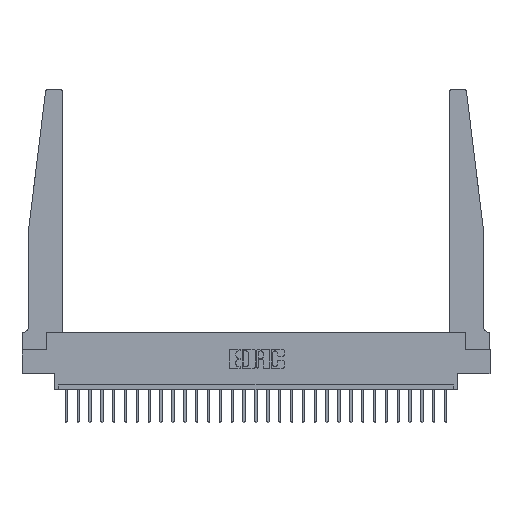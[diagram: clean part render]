
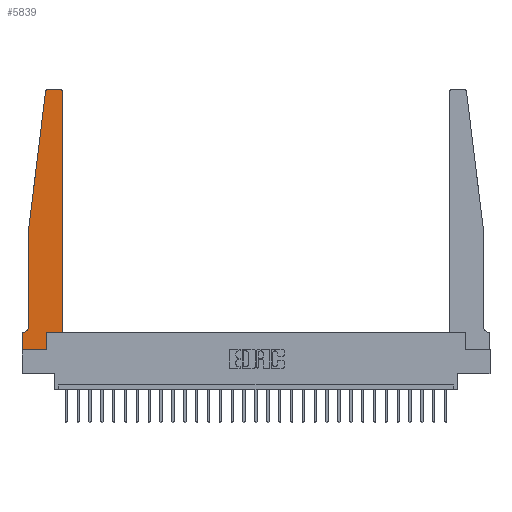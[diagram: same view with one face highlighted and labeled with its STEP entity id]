
A CAD part, top view. The second image highlights one B-rep face of the part: STEP entity #5839.
In plain terms, the highlighted planar face has unit normal (0, 0, 1).
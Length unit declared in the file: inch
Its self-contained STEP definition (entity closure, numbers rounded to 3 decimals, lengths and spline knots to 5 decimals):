
#637 = VERTEX_POINT ( 'NONE', #10416 ) ;
#946 = VERTEX_POINT ( 'NONE', #3312 ) ;
#1009 = CARTESIAN_POINT ( 'NONE',  ( 0.425, 0.18, 0.37 ) ) ;
#1124 = AXIS2_PLACEMENT_3D ( 'NONE', #7279, #9356, #19669 ) ;
#1316 = LINE ( 'NONE', #21824, #3554 ) ;
#1574 = DIRECTION ( 'NONE',  ( -1., 0., 0. ) ) ;
#1667 = EDGE_CURVE ( 'NONE', #16002, #22770, #25779, .T. ) ;
#1725 = CARTESIAN_POINT ( 'NONE',  ( 0., 0., 0.37 ) ) ;
#1814 = CARTESIAN_POINT ( 'NONE',  ( 0.2605, 0.18, 0.37 ) ) ;
#1879 = CARTESIAN_POINT ( 'NONE',  ( 0.27653, 2.75, 0.37 ) ) ;
#2254 = AXIS2_PLACEMENT_3D ( 'NONE', #18220, #24083, #1574 ) ;
#3105 = ORIENTED_EDGE ( 'NONE', *, *, #24069, .T. ) ;
#3312 = CARTESIAN_POINT ( 'NONE',  ( 0., 0.1875, 0.37 ) ) ;
#3509 = CIRCLE ( 'NONE', #10659, 0.03 ) ;
#3554 = VECTOR ( 'NONE', #13982, 39.37008 ) ;
#3640 = CARTESIAN_POINT ( 'NONE',  ( 0.065, 1.25, 0.37 ) ) ;
#3657 = VECTOR ( 'NONE', #10116, 39.37008 ) ;
#4074 = VECTOR ( 'NONE', #10125, 39.37008 ) ;
#4075 = CARTESIAN_POINT ( 'NONE',  ( 0.395, 2.75, 0.37 ) ) ;
#4081 = DIRECTION ( 'NONE',  ( 0., -1., 0. ) ) ;
#4325 = ORIENTED_EDGE ( 'NONE', *, *, #22656, .T. ) ;
#4931 = EDGE_CURVE ( 'NONE', #637, #23798, #25307, .T. ) ;
#5839 = ADVANCED_FACE ( 'NONE', ( #18187 ), #21760, .T. ) ;
#6051 = LINE ( 'NONE', #3640, #24047 ) ;
#6699 = VERTEX_POINT ( 'NONE', #6936 ) ;
#6936 = CARTESIAN_POINT ( 'NONE',  ( 0., 0., 0.37 ) ) ;
#7279 = CARTESIAN_POINT ( 'NONE',  ( 0., 0.1875, 0.37 ) ) ;
#7726 = DIRECTION ( 'NONE',  ( -0.122, -0.992, 0. ) ) ;
#7737 = AXIS2_PLACEMENT_3D ( 'NONE', #23165, #12834, #21101 ) ;
#8115 = ORIENTED_EDGE ( 'NONE', *, *, #17398, .T. ) ;
#8948 = VECTOR ( 'NONE', #19988, 39.37008 ) ;
#9356 = DIRECTION ( 'NONE',  ( 0., 0., 1. ) ) ;
#9669 = CARTESIAN_POINT ( 'NONE',  ( 0.2605, 0.18, 0.37 ) ) ;
#10116 = DIRECTION ( 'NONE',  ( 1., 0., 0. ) ) ;
#10125 = DIRECTION ( 'NONE',  ( 1., 0., 0. ) ) ;
#10416 = CARTESIAN_POINT ( 'NONE',  ( 0.2605, 0., 0.37 ) ) ;
#10659 = AXIS2_PLACEMENT_3D ( 'NONE', #15526, #17858, #11392 ) ;
#10714 = DIRECTION ( 'NONE',  ( 0., -1., 0. ) ) ;
#11392 = DIRECTION ( 'NONE',  ( 1., 0., 0. ) ) ;
#11589 = EDGE_CURVE ( 'NONE', #946, #6699, #17667, .T. ) ;
#12619 = EDGE_CURVE ( 'NONE', #6699, #637, #15049, .T. ) ;
#12621 = LINE ( 'NONE', #21473, #13282 ) ;
#12629 = ORIENTED_EDGE ( 'NONE', *, *, #1667, .T. ) ;
#12646 = VERTEX_POINT ( 'NONE', #4075 ) ;
#12834 = DIRECTION ( 'NONE',  ( 0., 0., 1. ) ) ;
#13282 = VECTOR ( 'NONE', #25388, 39.37008 ) ;
#13333 = ORIENTED_EDGE ( 'NONE', *, *, #25002, .T. ) ;
#13612 = ORIENTED_EDGE ( 'NONE', *, *, #12619, .T. ) ;
#13982 = DIRECTION ( 'NONE',  ( -1., 0., 0. ) ) ;
#14077 = CARTESIAN_POINT ( 'NONE',  ( 0.425, 2.72, 0.37 ) ) ;
#14176 = CARTESIAN_POINT ( 'NONE',  ( 0.24675, 2.72367, 0.37 ) ) ;
#14273 = VECTOR ( 'NONE', #19363, 39.37008 ) ;
#15049 = LINE ( 'NONE', #1725, #4074 ) ;
#15171 = VERTEX_POINT ( 'NONE', #1879 ) ;
#15319 = ORIENTED_EDGE ( 'NONE', *, *, #11589, .T. ) ;
#15526 = CARTESIAN_POINT ( 'NONE',  ( 0.27653, 2.72, 0.37 ) ) ;
#15672 = EDGE_CURVE ( 'NONE', #12646, #15171, #24545, .T. ) ;
#16002 = VERTEX_POINT ( 'NONE', #24972 ) ;
#16505 = EDGE_CURVE ( 'NONE', #18593, #16002, #20683, .T. ) ;
#16506 = CARTESIAN_POINT ( 'NONE',  ( 0.065, 1.25, 0.37 ) ) ;
#16660 = VERTEX_POINT ( 'NONE', #14176 ) ;
#16714 = ORIENTED_EDGE ( 'NONE', *, *, #23698, .T. ) ;
#17202 = CARTESIAN_POINT ( 'NONE',  ( 0., 0., 0.37 ) ) ;
#17398 = EDGE_CURVE ( 'NONE', #24133, #25622, #12621, .T. ) ;
#17667 = LINE ( 'NONE', #17202, #23797 ) ;
#17858 = DIRECTION ( 'NONE',  ( 0., 0., 1. ) ) ;
#17925 = ORIENTED_EDGE ( 'NONE', *, *, #16505, .T. ) ;
#18187 = FACE_OUTER_BOUND ( 'NONE', #18972, .T. ) ;
#18220 = CARTESIAN_POINT ( 'NONE',  ( 0.015, 0.2375, 0.37 ) ) ;
#18593 = VERTEX_POINT ( 'NONE', #23025 ) ;
#18972 = EDGE_LOOP ( 'NONE', ( #23665, #16714, #13333, #17925, #12629, #4325, #15319, #13612, #23908, #20509, #8115, #3105 ) ) ;
#19085 = VECTOR ( 'NONE', #4081, 39.37008 ) ;
#19363 = DIRECTION ( 'NONE',  ( -1., 0., 0. ) ) ;
#19669 = DIRECTION ( 'NONE',  ( 1., 0., 0. ) ) ;
#19988 = DIRECTION ( 'NONE',  ( 0., 1., 0. ) ) ;
#20351 = CARTESIAN_POINT ( 'NONE',  ( 0.015, 0.1875, 0.37 ) ) ;
#20509 = ORIENTED_EDGE ( 'NONE', *, *, #20860, .T. ) ;
#20683 = LINE ( 'NONE', #16506, #19085 ) ;
#20860 = EDGE_CURVE ( 'NONE', #23798, #24133, #23966, .T. ) ;
#21101 = DIRECTION ( 'NONE',  ( 1., 0., 0. ) ) ;
#21473 = CARTESIAN_POINT ( 'NONE',  ( 0.425, 0.18, 0.37 ) ) ;
#21624 = CARTESIAN_POINT ( 'NONE',  ( 0.25, 2.75, 0.37 ) ) ;
#21760 = PLANE ( 'NONE',  #1124 ) ;
#21824 = CARTESIAN_POINT ( 'NONE',  ( 0.065, 0.1875, 0.37 ) ) ;
#22656 = EDGE_CURVE ( 'NONE', #22770, #946, #1316, .T. ) ;
#22770 = VERTEX_POINT ( 'NONE', #20351 ) ;
#23025 = CARTESIAN_POINT ( 'NONE',  ( 0.065, 1.25, 0.37 ) ) ;
#23165 = CARTESIAN_POINT ( 'NONE',  ( 0.395, 2.72, 0.37 ) ) ;
#23665 = ORIENTED_EDGE ( 'NONE', *, *, #15672, .T. ) ;
#23698 = EDGE_CURVE ( 'NONE', #15171, #16660, #3509, .T. ) ;
#23797 = VECTOR ( 'NONE', #10714, 39.37008 ) ;
#23798 = VERTEX_POINT ( 'NONE', #1814 ) ;
#23908 = ORIENTED_EDGE ( 'NONE', *, *, #4931, .T. ) ;
#23966 = LINE ( 'NONE', #24653, #3657 ) ;
#24047 = VECTOR ( 'NONE', #7726, 39.37008 ) ;
#24069 = EDGE_CURVE ( 'NONE', #25622, #12646, #25676, .T. ) ;
#24083 = DIRECTION ( 'NONE',  ( 0., 0., -1. ) ) ;
#24133 = VERTEX_POINT ( 'NONE', #1009 ) ;
#24545 = LINE ( 'NONE', #21624, #14273 ) ;
#24653 = CARTESIAN_POINT ( 'NONE',  ( 0.425, 0.18, 0.37 ) ) ;
#24972 = CARTESIAN_POINT ( 'NONE',  ( 0.065, 0.2375, 0.37 ) ) ;
#25002 = EDGE_CURVE ( 'NONE', #16660, #18593, #6051, .T. ) ;
#25307 = LINE ( 'NONE', #9669, #8948 ) ;
#25388 = DIRECTION ( 'NONE',  ( 0., 1., 0. ) ) ;
#25622 = VERTEX_POINT ( 'NONE', #14077 ) ;
#25676 = CIRCLE ( 'NONE', #7737, 0.03 ) ;
#25779 = CIRCLE ( 'NONE', #2254, 0.05 ) ;
